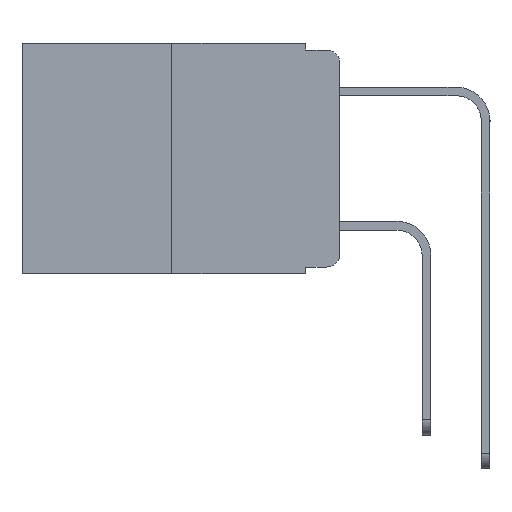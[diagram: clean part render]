
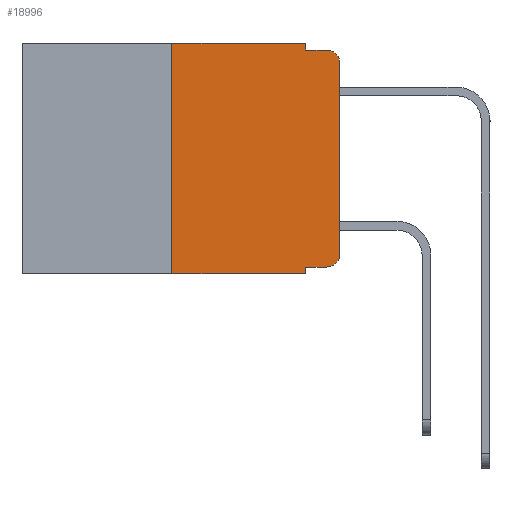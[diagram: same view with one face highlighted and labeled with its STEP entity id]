
A CAD part, left-side view. The second image highlights one B-rep face of the part: STEP entity #18996.
In plain terms, the highlighted planar face has unit normal (-1, 0, 0).
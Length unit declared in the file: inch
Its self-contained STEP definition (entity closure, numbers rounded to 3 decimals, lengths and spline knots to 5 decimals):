
#115 = CARTESIAN_POINT ( 'NONE',  ( 0., 0.473, 0. ) ) ;
#472 = LINE ( 'NONE', #10706, #12594 ) ;
#1018 = VECTOR ( 'NONE', #3748, 39.37008 ) ;
#1051 = CARTESIAN_POINT ( 'NONE',  ( 0., 0.051, 0. ) ) ;
#1099 = ORIENTED_EDGE ( 'NONE', *, *, #8993, .T. ) ;
#2018 = VERTEX_POINT ( 'NONE', #5408 ) ;
#2078 = VECTOR ( 'NONE', #2870, 39.37008 ) ;
#2406 = CARTESIAN_POINT ( 'NONE',  ( 0., 0.473, 0. ) ) ;
#2418 = CARTESIAN_POINT ( 'NONE',  ( 0., 0., 0. ) ) ;
#2542 = CARTESIAN_POINT ( 'NONE',  ( 0., 0.02, -0.333 ) ) ;
#2573 = LINE ( 'NONE', #10695, #2078 ) ;
#2614 = CARTESIAN_POINT ( 'NONE',  ( 0., 0.25, -0.343 ) ) ;
#2691 = CARTESIAN_POINT ( 'NONE',  ( 0., 0.051, -0.01 ) ) ;
#2870 = DIRECTION ( 'NONE',  ( 0., -1., 0. ) ) ;
#2954 = CARTESIAN_POINT ( 'NONE',  ( 0., 0., -0.03 ) ) ;
#3340 = ORIENTED_EDGE ( 'NONE', *, *, #7692, .F. ) ;
#3411 = EDGE_CURVE ( 'NONE', #14745, #14384, #472, .T. ) ;
#3487 = CARTESIAN_POINT ( 'NONE',  ( 0., 0.02, -0.313 ) ) ;
#3748 = DIRECTION ( 'NONE',  ( 0., -1., 0. ) ) ;
#3815 = ORIENTED_EDGE ( 'NONE', *, *, #3411, .F. ) ;
#4078 = DIRECTION ( 'NONE',  ( 0., -1., 0. ) ) ;
#4399 = DIRECTION ( 'NONE',  ( 0., 0., -1. ) ) ;
#4523 = VERTEX_POINT ( 'NONE', #2954 ) ;
#4593 = CARTESIAN_POINT ( 'NONE',  ( 0., 0.051, 0. ) ) ;
#5157 = DIRECTION ( 'NONE',  ( 0., 0., -1. ) ) ;
#5408 = CARTESIAN_POINT ( 'NONE',  ( 0., 0.02, -0.01 ) ) ;
#5458 = LINE ( 'NONE', #7488, #17107 ) ;
#5600 = CIRCLE ( 'NONE', #12169, 0.02 ) ;
#5894 = CARTESIAN_POINT ( 'NONE',  ( 0., 0.051, -0.333 ) ) ;
#6114 = VECTOR ( 'NONE', #10274, 39.37008 ) ;
#6549 = FACE_OUTER_BOUND ( 'NONE', #18941, .T. ) ;
#6594 = VERTEX_POINT ( 'NONE', #4593 ) ;
#6833 = ORIENTED_EDGE ( 'NONE', *, *, #13158, .T. ) ;
#6980 = CARTESIAN_POINT ( 'NONE',  ( 0., 0.051, -0.01 ) ) ;
#7056 = CIRCLE ( 'NONE', #14946, 0.02 ) ;
#7464 = DIRECTION ( 'NONE',  ( 0., -1., 0. ) ) ;
#7488 = CARTESIAN_POINT ( 'NONE',  ( 0., 0.051, 0. ) ) ;
#7692 = EDGE_CURVE ( 'NONE', #6594, #12902, #5458, .T. ) ;
#7741 = VECTOR ( 'NONE', #4399, 39.37008 ) ;
#8210 = EDGE_CURVE ( 'NONE', #14384, #6594, #16621, .T. ) ;
#8296 = DIRECTION ( 'NONE',  ( 1., 0., 0. ) ) ;
#8568 = ORIENTED_EDGE ( 'NONE', *, *, #11126, .T. ) ;
#8590 = LINE ( 'NONE', #6980, #1018 ) ;
#8622 = VECTOR ( 'NONE', #4078, 39.37008 ) ;
#8993 = EDGE_CURVE ( 'NONE', #14745, #15017, #2573, .T. ) ;
#9351 = DIRECTION ( 'NONE',  ( -1., 0., 0. ) ) ;
#9743 = EDGE_CURVE ( 'NONE', #12902, #2018, #8590, .T. ) ;
#10274 = DIRECTION ( 'NONE',  ( 0., 0., 1. ) ) ;
#10578 = VERTEX_POINT ( 'NONE', #2542 ) ;
#10695 = CARTESIAN_POINT ( 'NONE',  ( 0., 0.473, -0.343 ) ) ;
#10706 = CARTESIAN_POINT ( 'NONE',  ( 0., 0.25, 0. ) ) ;
#10750 = EDGE_CURVE ( 'NONE', #4523, #2018, #5600, .T. ) ;
#10936 = CARTESIAN_POINT ( 'NONE',  ( 0., 0.051, -0.333 ) ) ;
#11126 = EDGE_CURVE ( 'NONE', #13020, #10578, #14658, .T. ) ;
#11297 = CARTESIAN_POINT ( 'NONE',  ( 0., 0.051, -0.343 ) ) ;
#11632 = ORIENTED_EDGE ( 'NONE', *, *, #12789, .T. ) ;
#12124 = DIRECTION ( 'NONE',  ( 0., 0., -1. ) ) ;
#12169 = AXIS2_PLACEMENT_3D ( 'NONE', #18309, #9351, #19757 ) ;
#12594 = VECTOR ( 'NONE', #14933, 39.37008 ) ;
#12789 = EDGE_CURVE ( 'NONE', #17936, #4523, #17694, .T. ) ;
#12902 = VERTEX_POINT ( 'NONE', #2691 ) ;
#13020 = VERTEX_POINT ( 'NONE', #10936 ) ;
#13158 = EDGE_CURVE ( 'NONE', #10578, #17936, #7056, .T. ) ;
#13376 = AXIS2_PLACEMENT_3D ( 'NONE', #115, #8296, #18749 ) ;
#14161 = EDGE_CURVE ( 'NONE', #13020, #15017, #19644, .T. ) ;
#14162 = ORIENTED_EDGE ( 'NONE', *, *, #9743, .F. ) ;
#14298 = DIRECTION ( 'NONE',  ( -1., 0., 0. ) ) ;
#14301 = PLANE ( 'NONE',  #13376 ) ;
#14384 = VERTEX_POINT ( 'NONE', #18571 ) ;
#14563 = ORIENTED_EDGE ( 'NONE', *, *, #14161, .F. ) ;
#14638 = ORIENTED_EDGE ( 'NONE', *, *, #10750, .T. ) ;
#14658 = LINE ( 'NONE', #5894, #15149 ) ;
#14745 = VERTEX_POINT ( 'NONE', #2614 ) ;
#14933 = DIRECTION ( 'NONE',  ( 0., 0., 1. ) ) ;
#14946 = AXIS2_PLACEMENT_3D ( 'NONE', #3487, #14298, #5157 ) ;
#15017 = VERTEX_POINT ( 'NONE', #11297 ) ;
#15149 = VECTOR ( 'NONE', #7464, 39.37008 ) ;
#15383 = ORIENTED_EDGE ( 'NONE', *, *, #8210, .F. ) ;
#16621 = LINE ( 'NONE', #2406, #8622 ) ;
#17107 = VECTOR ( 'NONE', #12124, 39.37008 ) ;
#17694 = LINE ( 'NONE', #2418, #6114 ) ;
#17936 = VERTEX_POINT ( 'NONE', #18841 ) ;
#18309 = CARTESIAN_POINT ( 'NONE',  ( 0., 0.02, -0.03 ) ) ;
#18571 = CARTESIAN_POINT ( 'NONE',  ( 0., 0.25, 0. ) ) ;
#18749 = DIRECTION ( 'NONE',  ( 0., 0., -1. ) ) ;
#18841 = CARTESIAN_POINT ( 'NONE',  ( 0., 0., -0.313 ) ) ;
#18941 = EDGE_LOOP ( 'NONE', ( #11632, #14638, #14162, #3340, #15383, #3815, #1099, #14563, #8568, #6833 ) ) ;
#18996 = ADVANCED_FACE ( 'NONE', ( #6549 ), #14301, .F. ) ;
#19644 = LINE ( 'NONE', #1051, #7741 ) ;
#19757 = DIRECTION ( 'NONE',  ( 0., 0., -1. ) ) ;
